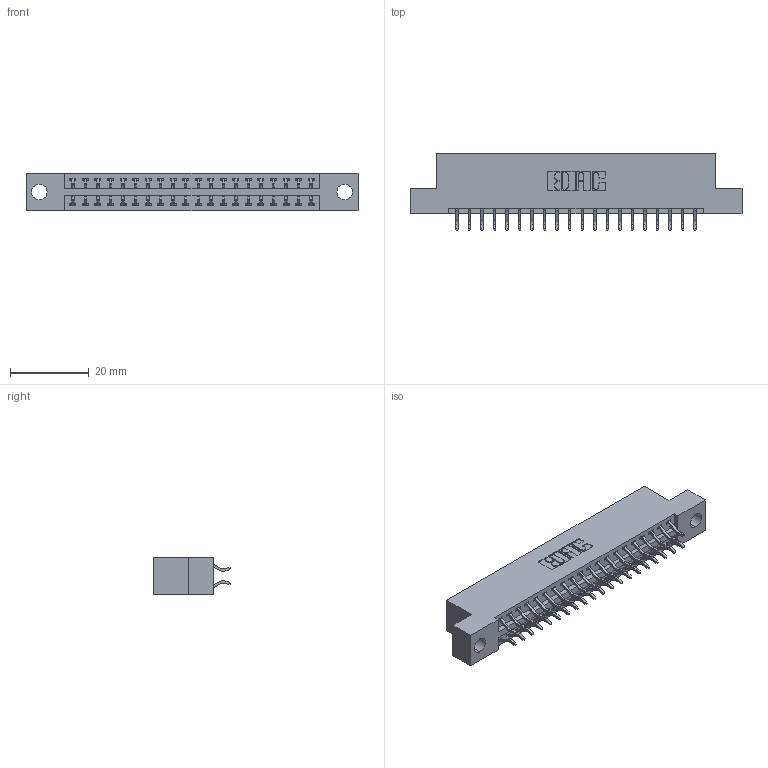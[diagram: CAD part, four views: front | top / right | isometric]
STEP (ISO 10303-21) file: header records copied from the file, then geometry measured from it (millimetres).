
FILE_DESCRIPTION (( 'STEP AP203' ), '1' );
FILE_NAME ('346-040-556-204.STEP', '2022-05-20T02:34:48', ( '' ), ( '' ), 'SwSTEP 2.0', 'SolidWorks 2020', '' );
FILE_SCHEMA (( 'CONFIG_CONTROL_DESIGN' ));
Length unit declared in the file: inch
Products named in the file (3): 346-040-556-204; 346 Part_Flush Mounting Lugs - 0.156 Dia-TH; 345-292-001_556 Tail
Assembly tree (41 placements, depth 2):
  346-040-556-204
    346 Part_Flush Mounting Lugs - 0.156 Dia-TH
    345-292-001_556 Tail  x40
Bounding box: 84.07 x 19.57 x 9.4 mm (x, y, z)
Volume: 7919.9 mm3; surface area: 10351.3 mm2
Topology: 41 solids, 41 shells, 2456 faces, 7285 edges, 4802 vertices
Faces by surface type: plane 1650, cylinder 806
Entity records: 16653 total; most frequent: CARTESIAN_POINT 2794, ORIENTED_EDGE 2714, DIRECTION 2501, EDGE_CURVE 1357, VECTOR 1137, LINE 1137, VERTEX_POINT 902, AXIS2_PLACEMENT_3D 682
